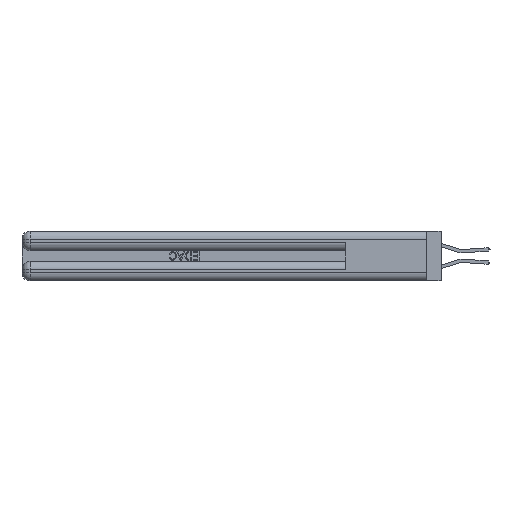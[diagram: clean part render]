
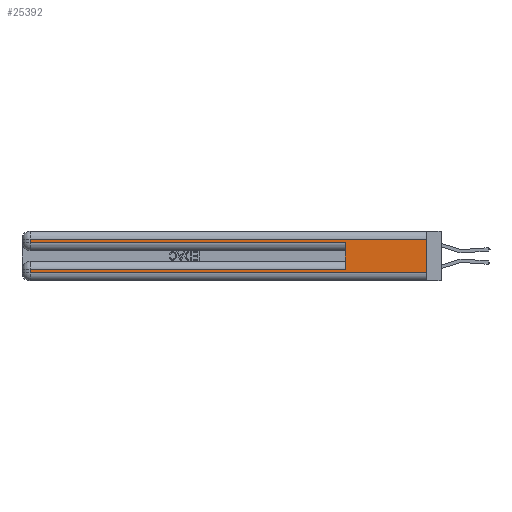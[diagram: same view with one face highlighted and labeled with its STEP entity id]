
A CAD part, left-side view. The second image highlights one B-rep face of the part: STEP entity #25392.
In plain terms, the highlighted planar face has unit normal (-1, 0, 0).
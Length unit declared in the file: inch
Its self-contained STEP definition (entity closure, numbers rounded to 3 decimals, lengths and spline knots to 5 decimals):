
#461 = DIRECTION ( 'NONE',  ( 1., 0., 0. ) ) ;
#953 = VERTEX_POINT ( 'NONE', #16739 ) ;
#1446 = AXIS2_PLACEMENT_3D ( 'NONE', #20893, #461, #24305 ) ;
#1941 = CARTESIAN_POINT ( 'NONE',  ( 0., 2.94, 0.085 ) ) ;
#2734 = ORIENTED_EDGE ( 'NONE', *, *, #10367, .T. ) ;
#3915 = VERTEX_POINT ( 'NONE', #5971 ) ;
#3921 = CARTESIAN_POINT ( 'NONE',  ( 0., 0., 0.31 ) ) ;
#4070 = VERTEX_POINT ( 'NONE', #16829 ) ;
#4292 = CARTESIAN_POINT ( 'NONE',  ( 0., 0., 0.085 ) ) ;
#5044 = VECTOR ( 'NONE', #35896, 39.37008 ) ;
#5603 = ORIENTED_EDGE ( 'NONE', *, *, #29642, .F. ) ;
#5971 = CARTESIAN_POINT ( 'NONE',  ( 0., 0.6, 0.085 ) ) ;
#8160 = DIRECTION ( 'NONE',  ( 0., 0., 1. ) ) ;
#8545 = VERTEX_POINT ( 'NONE', #31571 ) ;
#9614 = LINE ( 'NONE', #15166, #36386 ) ;
#9619 = CARTESIAN_POINT ( 'NONE',  ( 0., 0., 0.37 ) ) ;
#9863 = VERTEX_POINT ( 'NONE', #18741 ) ;
#9928 = VECTOR ( 'NONE', #18529, 39.37008 ) ;
#10367 = EDGE_CURVE ( 'NONE', #3915, #15963, #22146, .T. ) ;
#11215 = EDGE_CURVE ( 'NONE', #9863, #28372, #31996, .T. ) ;
#13252 = EDGE_CURVE ( 'NONE', #4070, #953, #36465, .T. ) ;
#14185 = VECTOR ( 'NONE', #36459, 39.37008 ) ;
#14272 = DIRECTION ( 'NONE',  ( 0., 0., -1. ) ) ;
#15166 = CARTESIAN_POINT ( 'NONE',  ( 0., 0.6, 0.145 ) ) ;
#15963 = VERTEX_POINT ( 'NONE', #1941 ) ;
#16114 = EDGE_CURVE ( 'NONE', #35144, #4070, #42516, .T. ) ;
#16739 = CARTESIAN_POINT ( 'NONE',  ( 0., 2.94, 0.285 ) ) ;
#16829 = CARTESIAN_POINT ( 'NONE',  ( 0., 2.94, 0.31 ) ) ;
#17499 = PLANE ( 'NONE',  #1446 ) ;
#17911 = LINE ( 'NONE', #38484, #9928 ) ;
#18023 = DIRECTION ( 'NONE',  ( 0., 1., 0. ) ) ;
#18529 = DIRECTION ( 'NONE',  ( 0., 0., -1. ) ) ;
#18729 = VECTOR ( 'NONE', #14272, 39.37008 ) ;
#18741 = CARTESIAN_POINT ( 'NONE',  ( 0., 2.94, 0.06 ) ) ;
#19186 = DIRECTION ( 'NONE',  ( 0., -1., 0. ) ) ;
#19389 = CARTESIAN_POINT ( 'NONE',  ( 0., 0., 0.31 ) ) ;
#19558 = ORIENTED_EDGE ( 'NONE', *, *, #42604, .T. ) ;
#20893 = CARTESIAN_POINT ( 'NONE',  ( 0., 0., 0.37 ) ) ;
#21242 = FACE_OUTER_BOUND ( 'NONE', #31410, .T. ) ;
#22146 = LINE ( 'NONE', #4292, #30009 ) ;
#23277 = ORIENTED_EDGE ( 'NONE', *, *, #11215, .T. ) ;
#23715 = ORIENTED_EDGE ( 'NONE', *, *, #13252, .T. ) ;
#24021 = EDGE_CURVE ( 'NONE', #3915, #8545, #9614, .T. ) ;
#24305 = DIRECTION ( 'NONE',  ( 0., 0., -1. ) ) ;
#24313 = DIRECTION ( 'NONE',  ( 0., 1., 0. ) ) ;
#24329 = CARTESIAN_POINT ( 'NONE',  ( 0., 2.94, 0.37 ) ) ;
#24902 = VECTOR ( 'NONE', #24313, 39.37008 ) ;
#25392 = ADVANCED_FACE ( 'NONE', ( #21242 ), #17499, .F. ) ;
#26047 = CARTESIAN_POINT ( 'NONE',  ( 0., 0., 0.06 ) ) ;
#26318 = LINE ( 'NONE', #9619, #14185 ) ;
#27030 = ORIENTED_EDGE ( 'NONE', *, *, #16114, .T. ) ;
#28372 = VERTEX_POINT ( 'NONE', #43051 ) ;
#29642 = EDGE_CURVE ( 'NONE', #35144, #28372, #26318, .T. ) ;
#30009 = VECTOR ( 'NONE', #18023, 39.37008 ) ;
#31410 = EDGE_LOOP ( 'NONE', ( #5603, #27030, #23715, #35633, #41330, #2734, #19558, #23277 ) ) ;
#31571 = CARTESIAN_POINT ( 'NONE',  ( 0., 0.6, 0.285 ) ) ;
#31996 = LINE ( 'NONE', #26047, #5044 ) ;
#35144 = VERTEX_POINT ( 'NONE', #19389 ) ;
#35633 = ORIENTED_EDGE ( 'NONE', *, *, #39553, .T. ) ;
#35896 = DIRECTION ( 'NONE',  ( 0., -1., 0. ) ) ;
#36386 = VECTOR ( 'NONE', #8160, 39.37008 ) ;
#36459 = DIRECTION ( 'NONE',  ( 0., 0., -1. ) ) ;
#36465 = LINE ( 'NONE', #24329, #18729 ) ;
#38484 = CARTESIAN_POINT ( 'NONE',  ( 0., 2.94, 0.37 ) ) ;
#39127 = CARTESIAN_POINT ( 'NONE',  ( 0., 0., 0.285 ) ) ;
#39553 = EDGE_CURVE ( 'NONE', #953, #8545, #42474, .T. ) ;
#41330 = ORIENTED_EDGE ( 'NONE', *, *, #24021, .F. ) ;
#41428 = VECTOR ( 'NONE', #19186, 39.37008 ) ;
#42474 = LINE ( 'NONE', #39127, #41428 ) ;
#42516 = LINE ( 'NONE', #3921, #24902 ) ;
#42604 = EDGE_CURVE ( 'NONE', #15963, #9863, #17911, .T. ) ;
#43051 = CARTESIAN_POINT ( 'NONE',  ( 0., 0., 0.06 ) ) ;
